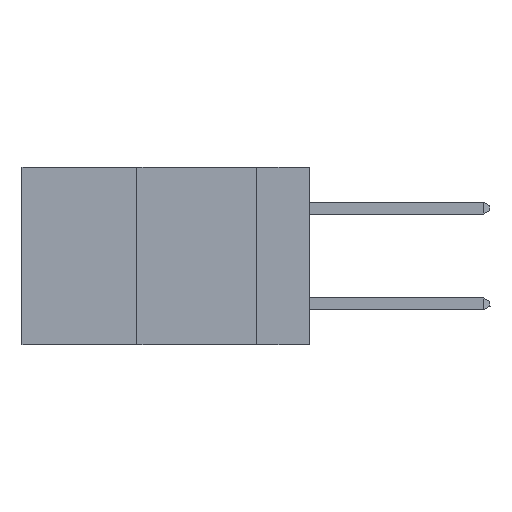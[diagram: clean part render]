
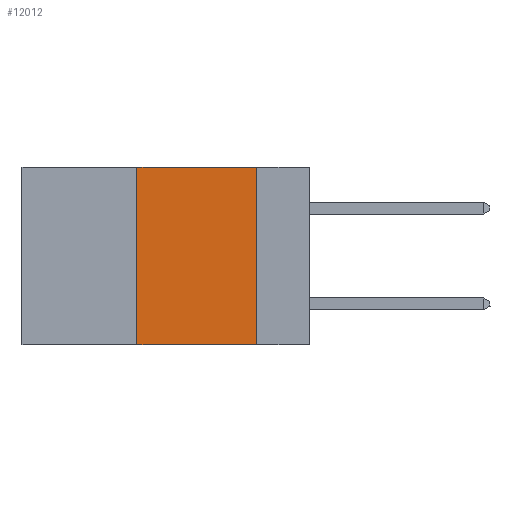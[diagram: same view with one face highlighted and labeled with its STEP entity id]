
A CAD part, left-side view. The second image highlights one B-rep face of the part: STEP entity #12012.
In plain terms, the highlighted planar face has unit normal (-1, 0, 0).
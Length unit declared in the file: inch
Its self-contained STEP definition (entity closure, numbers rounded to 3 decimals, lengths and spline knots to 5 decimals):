
#150 = VECTOR ( 'NONE', #13058, 39.37008 ) ;
#214 = LINE ( 'NONE', #4925, #2103 ) ;
#505 = VECTOR ( 'NONE', #6232, 39.37008 ) ;
#2103 = VECTOR ( 'NONE', #23874, 39.37008 ) ;
#2132 = CARTESIAN_POINT ( 'NONE',  ( 0., 0.11, 0. ) ) ;
#3870 = VERTEX_POINT ( 'NONE', #2132 ) ;
#4925 = CARTESIAN_POINT ( 'NONE',  ( 0., 0.11, 0. ) ) ;
#5530 = DIRECTION ( 'NONE',  ( 0., -1., 0. ) ) ;
#6135 = FACE_OUTER_BOUND ( 'NONE', #11458, .T. ) ;
#6232 = DIRECTION ( 'NONE',  ( 0., -1., 0. ) ) ;
#6577 = LINE ( 'NONE', #10981, #505 ) ;
#6746 = CARTESIAN_POINT ( 'NONE',  ( 0., 0.36, -0.37 ) ) ;
#8128 = EDGE_CURVE ( 'NONE', #8611, #3870, #6577, .T. ) ;
#8157 = EDGE_CURVE ( 'NONE', #27286, #8611, #16709, .T. ) ;
#8611 = VERTEX_POINT ( 'NONE', #19324 ) ;
#10981 = CARTESIAN_POINT ( 'NONE',  ( 0., 0.6, 0. ) ) ;
#11458 = EDGE_LOOP ( 'NONE', ( #23367, #19674, #29101, #24517 ) ) ;
#12012 = ADVANCED_FACE ( 'NONE', ( #6135 ), #22936, .F. ) ;
#13058 = DIRECTION ( 'NONE',  ( 0., 0., 1. ) ) ;
#16709 = LINE ( 'NONE', #22957, #150 ) ;
#18247 = CARTESIAN_POINT ( 'NONE',  ( 0., 0.6, 0. ) ) ;
#19324 = CARTESIAN_POINT ( 'NONE',  ( 0., 0.36, 0. ) ) ;
#19674 = ORIENTED_EDGE ( 'NONE', *, *, #8128, .F. ) ;
#19894 = CARTESIAN_POINT ( 'NONE',  ( 0., 0.6, -0.37 ) ) ;
#20919 = VECTOR ( 'NONE', #5530, 39.37008 ) ;
#21949 = CARTESIAN_POINT ( 'NONE',  ( 0., 0.11, -0.37 ) ) ;
#22663 = VERTEX_POINT ( 'NONE', #21949 ) ;
#22824 = DIRECTION ( 'NONE',  ( 0., 0., -1. ) ) ;
#22936 = PLANE ( 'NONE',  #24206 ) ;
#22957 = CARTESIAN_POINT ( 'NONE',  ( 0., 0.36, 0. ) ) ;
#23367 = ORIENTED_EDGE ( 'NONE', *, *, #24765, .F. ) ;
#23874 = DIRECTION ( 'NONE',  ( 0., 0., -1. ) ) ;
#24206 = AXIS2_PLACEMENT_3D ( 'NONE', #18247, #27876, #22824 ) ;
#24517 = ORIENTED_EDGE ( 'NONE', *, *, #29492, .T. ) ;
#24765 = EDGE_CURVE ( 'NONE', #3870, #22663, #214, .T. ) ;
#27286 = VERTEX_POINT ( 'NONE', #6746 ) ;
#27876 = DIRECTION ( 'NONE',  ( 1., 0., 0. ) ) ;
#29101 = ORIENTED_EDGE ( 'NONE', *, *, #8157, .F. ) ;
#29107 = LINE ( 'NONE', #19894, #20919 ) ;
#29492 = EDGE_CURVE ( 'NONE', #27286, #22663, #29107, .T. ) ;
